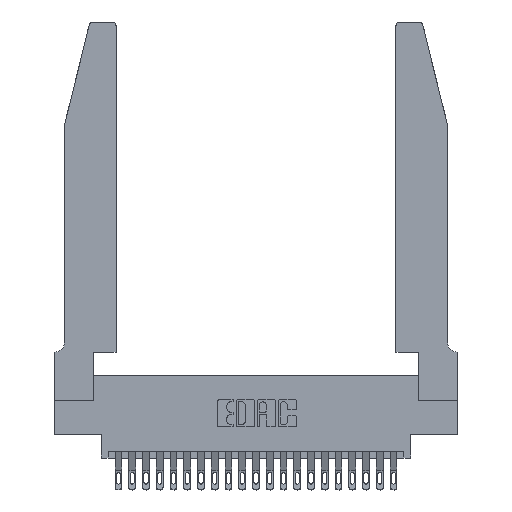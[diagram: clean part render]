
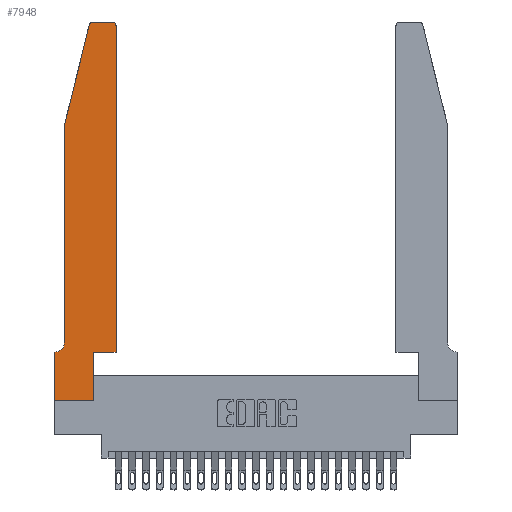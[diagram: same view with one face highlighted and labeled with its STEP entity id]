
A CAD part, top view. The second image highlights one B-rep face of the part: STEP entity #7948.
In plain terms, the highlighted planar face has unit normal (0, 0, 1).
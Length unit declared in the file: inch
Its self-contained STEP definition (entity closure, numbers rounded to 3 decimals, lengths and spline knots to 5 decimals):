
#11 = EDGE_CURVE ( 'NONE', #750, #20873, #5422, .T. ) ;
#488 = LINE ( 'NONE', #24356, #11038 ) ;
#563 = EDGE_CURVE ( 'NONE', #23996, #1440, #23530, .T. ) ;
#690 = ORIENTED_EDGE ( 'NONE', *, *, #1116, .T. ) ;
#750 = VERTEX_POINT ( 'NONE', #4415 ) ;
#818 = VERTEX_POINT ( 'NONE', #12224 ) ;
#915 = VECTOR ( 'NONE', #4966, 39.37008 ) ;
#963 = VECTOR ( 'NONE', #11166, 39.37008 ) ;
#1116 = EDGE_CURVE ( 'NONE', #22773, #2719, #13241, .T. ) ;
#1440 = VERTEX_POINT ( 'NONE', #13950 ) ;
#1717 = DIRECTION ( 'NONE',  ( 0., 0., 1. ) ) ;
#1801 = VECTOR ( 'NONE', #8556, 39.37008 ) ;
#2078 = EDGE_CURVE ( 'NONE', #818, #750, #4097, .T. ) ;
#2110 = CARTESIAN_POINT ( 'NONE',  ( 0., 0., 0.37 ) ) ;
#2141 = CARTESIAN_POINT ( 'NONE',  ( 0., 0.35, 0.37 ) ) ;
#2719 = VERTEX_POINT ( 'NONE', #10022 ) ;
#2746 = AXIS2_PLACEMENT_3D ( 'NONE', #13639, #1717, #23273 ) ;
#3082 = EDGE_CURVE ( 'NONE', #5114, #818, #15166, .T. ) ;
#4097 = LINE ( 'NONE', #2110, #18629 ) ;
#4135 = DIRECTION ( 'NONE',  ( 1., 0., 0. ) ) ;
#4415 = CARTESIAN_POINT ( 'NONE',  ( 0.2865, 0., 0.37 ) ) ;
#4595 = ORIENTED_EDGE ( 'NONE', *, *, #10513, .T. ) ;
#4692 = EDGE_CURVE ( 'NONE', #21996, #5114, #21967, .T. ) ;
#4827 = VECTOR ( 'NONE', #11560, 39.37008 ) ;
#4945 = CARTESIAN_POINT ( 'NONE',  ( 0.284, 2.75, 0.37 ) ) ;
#4966 = DIRECTION ( 'NONE',  ( 1., 0., 0. ) ) ;
#5114 = VERTEX_POINT ( 'NONE', #2141 ) ;
#5245 = CARTESIAN_POINT ( 'NONE',  ( 0.2605, 2.75, 0.37 ) ) ;
#5330 = LINE ( 'NONE', #18221, #19766 ) ;
#5340 = DIRECTION ( 'NONE',  ( 0., -1., 0. ) ) ;
#5422 = LINE ( 'NONE', #5911, #4827 ) ;
#5567 = CIRCLE ( 'NONE', #20369, 0.07 ) ;
#5911 = CARTESIAN_POINT ( 'NONE',  ( 0.2865, 0.35, 0.37 ) ) ;
#6626 = CARTESIAN_POINT ( 'NONE',  ( 0.0755, 0.35, 0.37 ) ) ;
#7444 = VERTEX_POINT ( 'NONE', #9053 ) ;
#7650 = ORIENTED_EDGE ( 'NONE', *, *, #23719, .T. ) ;
#7735 = ORIENTED_EDGE ( 'NONE', *, *, #9018, .T. ) ;
#7948 = ADVANCED_FACE ( 'NONE', ( #18118 ), #9270, .T. ) ;
#8349 = ORIENTED_EDGE ( 'NONE', *, *, #2078, .T. ) ;
#8556 = DIRECTION ( 'NONE',  ( -1., 0., 0. ) ) ;
#9018 = EDGE_CURVE ( 'NONE', #1440, #15553, #11473, .T. ) ;
#9053 = CARTESIAN_POINT ( 'NONE',  ( 0.25487, 2.72718, 0.37 ) ) ;
#9270 = PLANE ( 'NONE',  #11283 ) ;
#9819 = DIRECTION ( 'NONE',  ( 0., 0., -1. ) ) ;
#10022 = CARTESIAN_POINT ( 'NONE',  ( 0.0755, 0.42, 0.37 ) ) ;
#10098 = EDGE_LOOP ( 'NONE', ( #7735, #15488, #7650, #690, #4595, #15431, #21152, #8349, #16404, #21826, #10368, #23655 ) ) ;
#10368 = ORIENTED_EDGE ( 'NONE', *, *, #21048, .T. ) ;
#10513 = EDGE_CURVE ( 'NONE', #2719, #21996, #5567, .T. ) ;
#11038 = VECTOR ( 'NONE', #13450, 39.37008 ) ;
#11166 = DIRECTION ( 'NONE',  ( -1., 0., 0. ) ) ;
#11200 = CARTESIAN_POINT ( 'NONE',  ( 0.0755, 2., 0.37 ) ) ;
#11216 = DIRECTION ( 'NONE',  ( 1., 0., 0. ) ) ;
#11283 = AXIS2_PLACEMENT_3D ( 'NONE', #14830, #22184, #11216 ) ;
#11328 = DIRECTION ( 'NONE',  ( 0., 0., 1. ) ) ;
#11441 = LINE ( 'NONE', #18190, #915 ) ;
#11473 = LINE ( 'NONE', #5245, #963 ) ;
#11560 = DIRECTION ( 'NONE',  ( 0., 1., 0. ) ) ;
#12155 = CARTESIAN_POINT ( 'NONE',  ( 0.2865, 0.35, 0.37 ) ) ;
#12224 = CARTESIAN_POINT ( 'NONE',  ( 0., 0., 0.37 ) ) ;
#12677 = VECTOR ( 'NONE', #5340, 39.37008 ) ;
#13062 = CARTESIAN_POINT ( 'NONE',  ( 0.0055, 0.35, 0.37 ) ) ;
#13241 = LINE ( 'NONE', #11200, #12677 ) ;
#13450 = DIRECTION ( 'NONE',  ( -0.239, -0.971, 0. ) ) ;
#13639 = CARTESIAN_POINT ( 'NONE',  ( 0.4205, 2.72, 0.37 ) ) ;
#13950 = CARTESIAN_POINT ( 'NONE',  ( 0.4205, 2.75, 0.37 ) ) ;
#14182 = CIRCLE ( 'NONE', #21373, 0.03 ) ;
#14830 = CARTESIAN_POINT ( 'NONE',  ( 0., 0.35, 0.37 ) ) ;
#15166 = LINE ( 'NONE', #18824, #23164 ) ;
#15431 = ORIENTED_EDGE ( 'NONE', *, *, #4692, .T. ) ;
#15488 = ORIENTED_EDGE ( 'NONE', *, *, #24272, .T. ) ;
#15553 = VERTEX_POINT ( 'NONE', #4945 ) ;
#16404 = ORIENTED_EDGE ( 'NONE', *, *, #11, .T. ) ;
#17812 = CARTESIAN_POINT ( 'NONE',  ( 0.0755, 2., 0.37 ) ) ;
#17910 = CARTESIAN_POINT ( 'NONE',  ( 0.4505, 2.72, 0.37 ) ) ;
#18118 = FACE_OUTER_BOUND ( 'NONE', #10098, .T. ) ;
#18190 = CARTESIAN_POINT ( 'NONE',  ( 0.4505, 0.35, 0.37 ) ) ;
#18221 = CARTESIAN_POINT ( 'NONE',  ( 0.4505, 0.35, 0.37 ) ) ;
#18629 = VECTOR ( 'NONE', #4135, 39.37008 ) ;
#18824 = CARTESIAN_POINT ( 'NONE',  ( 0., 0., 0.37 ) ) ;
#19766 = VECTOR ( 'NONE', #20058, 39.37008 ) ;
#20058 = DIRECTION ( 'NONE',  ( 0., 1., 0. ) ) ;
#20311 = VERTEX_POINT ( 'NONE', #23339 ) ;
#20369 = AXIS2_PLACEMENT_3D ( 'NONE', #20876, #9819, #22699 ) ;
#20663 = DIRECTION ( 'NONE',  ( 0., -1., 0. ) ) ;
#20873 = VERTEX_POINT ( 'NONE', #12155 ) ;
#20876 = CARTESIAN_POINT ( 'NONE',  ( 0.0055, 0.42, 0.37 ) ) ;
#21048 = EDGE_CURVE ( 'NONE', #20311, #23996, #5330, .T. ) ;
#21152 = ORIENTED_EDGE ( 'NONE', *, *, #3082, .T. ) ;
#21373 = AXIS2_PLACEMENT_3D ( 'NONE', #22278, #11328, #24106 ) ;
#21670 = EDGE_CURVE ( 'NONE', #20873, #20311, #11441, .T. ) ;
#21826 = ORIENTED_EDGE ( 'NONE', *, *, #21670, .T. ) ;
#21967 = LINE ( 'NONE', #6626, #1801 ) ;
#21996 = VERTEX_POINT ( 'NONE', #13062 ) ;
#22184 = DIRECTION ( 'NONE',  ( 0., 0., 1. ) ) ;
#22278 = CARTESIAN_POINT ( 'NONE',  ( 0.284, 2.72, 0.37 ) ) ;
#22699 = DIRECTION ( 'NONE',  ( -1., 0., 0. ) ) ;
#22773 = VERTEX_POINT ( 'NONE', #17812 ) ;
#23164 = VECTOR ( 'NONE', #20663, 39.37008 ) ;
#23273 = DIRECTION ( 'NONE',  ( 1., 0., 0. ) ) ;
#23339 = CARTESIAN_POINT ( 'NONE',  ( 0.4505, 0.35, 0.37 ) ) ;
#23530 = CIRCLE ( 'NONE', #2746, 0.03 ) ;
#23655 = ORIENTED_EDGE ( 'NONE', *, *, #563, .T. ) ;
#23719 = EDGE_CURVE ( 'NONE', #7444, #22773, #488, .T. ) ;
#23996 = VERTEX_POINT ( 'NONE', #17910 ) ;
#24106 = DIRECTION ( 'NONE',  ( 1., 0., 0. ) ) ;
#24272 = EDGE_CURVE ( 'NONE', #15553, #7444, #14182, .T. ) ;
#24356 = CARTESIAN_POINT ( 'NONE',  ( 0.0755, 2., 0.37 ) ) ;
